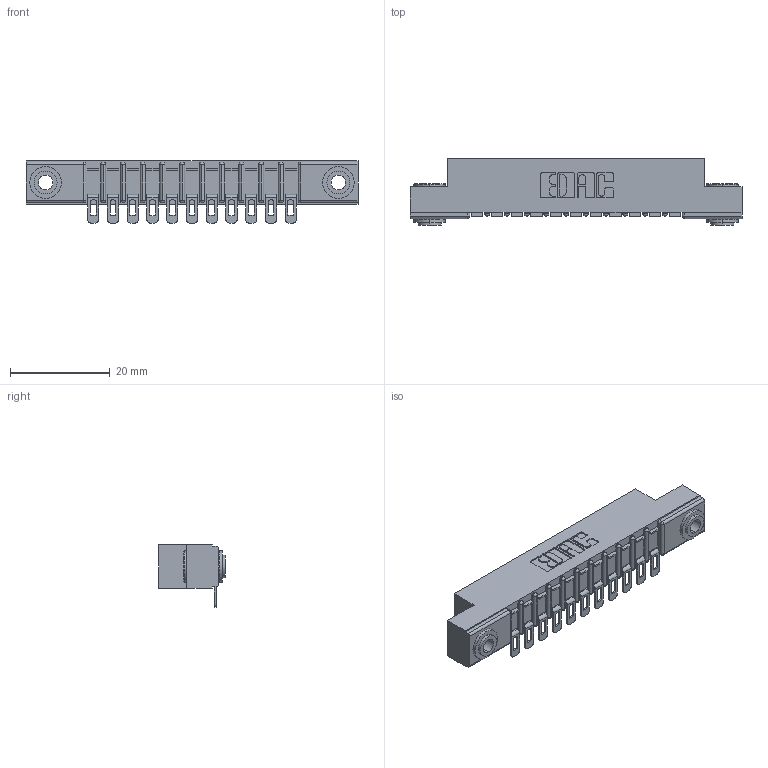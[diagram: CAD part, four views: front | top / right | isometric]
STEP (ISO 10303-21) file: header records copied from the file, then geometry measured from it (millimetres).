
FILE_DESCRIPTION (( 'STEP AP203' ), '1' );
FILE_NAME ('307-011-554-103.STEP', '2018-08-02T22:07:18', ( '' ), ( '' ), 'SwSTEP 2.0', 'SolidWorks 2016', '' );
FILE_SCHEMA (( 'CONFIG_CONTROL_DESIGN' ));
Length unit declared in the file: inch
Products named in the file (4): 307-290-002_554; 345-250-002_345-250-002-102; 307-011-554-103; 307 Part_.156 Dia Mounting Holes
Assembly tree (14 placements, depth 2):
  307-011-554-103
    307 Part_.156 Dia Mounting Holes
    307-290-002_554  x11
    345-250-002_345-250-002-102  x2
Bounding box: 66.6 x 13.36 x 12.52 mm (x, y, z)
Volume: 4396.2 mm3; surface area: 7673.6 mm2
Topology: 14 solids, 14 shells, 1073 faces, 3218 edges, 2108 vertices
Faces by surface type: plane 600, cylinder 441, sphere 24, cone 8
Entity records: 15282 total; most frequent: CARTESIAN_POINT 2551, ORIENTED_EDGE 2532, DIRECTION 2514, EDGE_CURVE 1266, LINE 940, VECTOR 940, VERTEX_POINT 824, AXIS2_PLACEMENT_3D 787
